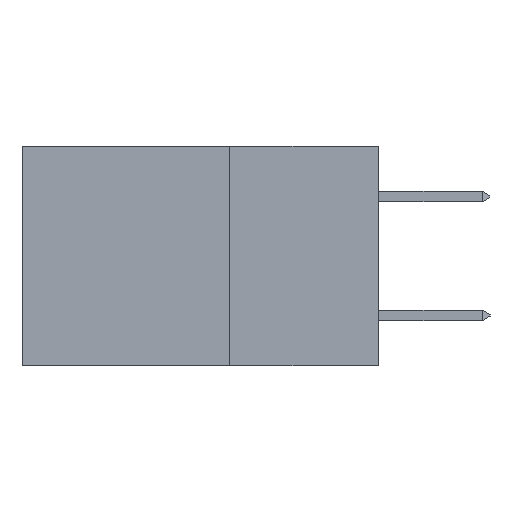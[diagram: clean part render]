
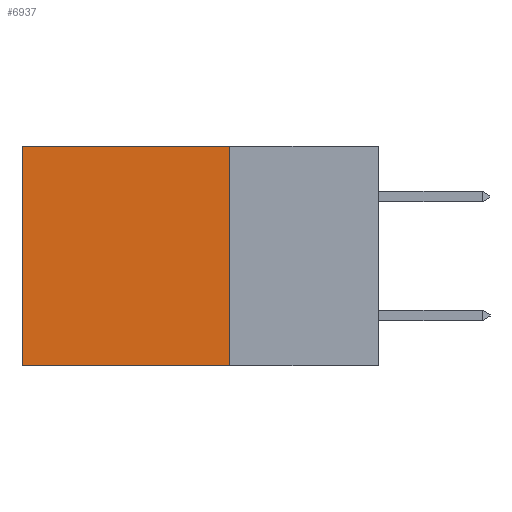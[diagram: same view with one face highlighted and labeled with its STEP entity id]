
A CAD part, left-side view. The second image highlights one B-rep face of the part: STEP entity #6937.
In plain terms, the highlighted planar face has unit normal (-1, 0, 0).
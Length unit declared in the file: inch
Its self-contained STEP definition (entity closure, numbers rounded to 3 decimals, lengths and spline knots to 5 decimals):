
#2730 = CARTESIAN_POINT ( 'NONE',  ( 0.2615, 0.25, -0.37 ) ) ;
#2866 = EDGE_CURVE ( 'NONE', #8574, #11687, #14195, .T. ) ;
#2990 = CARTESIAN_POINT ( 'NONE',  ( 0.2615, 0.6, 0. ) ) ;
#3348 = CARTESIAN_POINT ( 'NONE',  ( 0.2615, 0.25, -0.37 ) ) ;
#3720 = EDGE_CURVE ( 'NONE', #10272, #4022, #6028, .T. ) ;
#4022 = VERTEX_POINT ( 'NONE', #3348 ) ;
#4033 = DIRECTION ( 'NONE',  ( 0., 1., 0. ) ) ;
#4155 = CARTESIAN_POINT ( 'NONE',  ( 0.2615, 0.6, -0.37 ) ) ;
#4225 = DIRECTION ( 'NONE',  ( 0., 1., 0. ) ) ;
#4508 = VECTOR ( 'NONE', #4225, 39.37008 ) ;
#6028 = LINE ( 'NONE', #10438, #8451 ) ;
#6677 = ORIENTED_EDGE ( 'NONE', *, *, #3720, .F. ) ;
#6937 = ADVANCED_FACE ( 'NONE', ( #7945 ), #8180, .F. ) ;
#7213 = EDGE_LOOP ( 'NONE', ( #9075, #10134, #6677, #11285 ) ) ;
#7700 = AXIS2_PLACEMENT_3D ( 'NONE', #8312, #8098, #8026 ) ;
#7945 = FACE_OUTER_BOUND ( 'NONE', #7213, .T. ) ;
#8026 = DIRECTION ( 'NONE',  ( 0., 0., -1. ) ) ;
#8098 = DIRECTION ( 'NONE',  ( 1., 0., 0. ) ) ;
#8105 = VECTOR ( 'NONE', #11344, 39.37008 ) ;
#8180 = PLANE ( 'NONE',  #7700 ) ;
#8312 = CARTESIAN_POINT ( 'NONE',  ( 0.2615, 0.25, -0.37 ) ) ;
#8451 = VECTOR ( 'NONE', #10228, 39.37008 ) ;
#8574 = VERTEX_POINT ( 'NONE', #2990 ) ;
#9075 = ORIENTED_EDGE ( 'NONE', *, *, #2866, .T. ) ;
#10134 = ORIENTED_EDGE ( 'NONE', *, *, #13126, .F. ) ;
#10228 = DIRECTION ( 'NONE',  ( 0., 0., -1. ) ) ;
#10272 = VERTEX_POINT ( 'NONE', #14248 ) ;
#10438 = CARTESIAN_POINT ( 'NONE',  ( 0.2615, 0.25, -0.37 ) ) ;
#11148 = LINE ( 'NONE', #12458, #4508 ) ;
#11207 = CARTESIAN_POINT ( 'NONE',  ( 0.2615, 0.6, -0.37 ) ) ;
#11285 = ORIENTED_EDGE ( 'NONE', *, *, #13234, .T. ) ;
#11344 = DIRECTION ( 'NONE',  ( 0., 0., -1. ) ) ;
#11687 = VERTEX_POINT ( 'NONE', #4155 ) ;
#12253 = VECTOR ( 'NONE', #4033, 39.37008 ) ;
#12458 = CARTESIAN_POINT ( 'NONE',  ( 0.2615, 0.25, 0. ) ) ;
#13126 = EDGE_CURVE ( 'NONE', #4022, #11687, #13300, .T. ) ;
#13234 = EDGE_CURVE ( 'NONE', #10272, #8574, #11148, .T. ) ;
#13300 = LINE ( 'NONE', #2730, #12253 ) ;
#14195 = LINE ( 'NONE', #11207, #8105 ) ;
#14248 = CARTESIAN_POINT ( 'NONE',  ( 0.2615, 0.25, 0. ) ) ;
